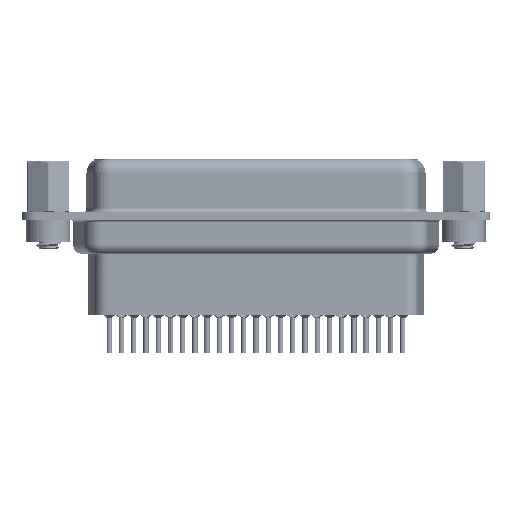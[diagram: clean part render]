
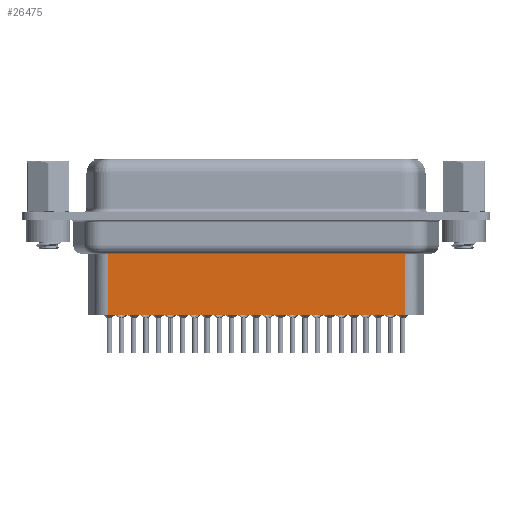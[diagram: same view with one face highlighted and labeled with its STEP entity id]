
A CAD part, front view. The second image highlights one B-rep face of the part: STEP entity #26475.
In plain terms, the highlighted planar face has unit normal (0, -1, 0).
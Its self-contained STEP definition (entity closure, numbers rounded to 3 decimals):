
#90 = CARTESIAN_POINT ( 'NONE',  ( 6.706, -3.5, -11.15 ) ) ;
#1557 = CARTESIAN_POINT ( 'NONE',  ( 6.706, -3.5, -3.1 ) ) ;
#2123 = LINE ( 'NONE', #7905, #11021 ) ;
#3071 = VECTOR ( 'NONE', #17312, 1000. ) ;
#3142 = CARTESIAN_POINT ( 'NONE',  ( 6.706, -3.5, -11.15 ) ) ;
#3190 = DIRECTION ( 'NONE',  ( 0., -1., 0. ) ) ;
#3309 = DIRECTION ( 'NONE',  ( -1., 0., 0. ) ) ;
#5667 = FACE_OUTER_BOUND ( 'NONE', #26028, .T. ) ;
#6197 = AXIS2_PLACEMENT_3D ( 'NONE', #15733, #3190, #30944 ) ;
#6871 = ORIENTED_EDGE ( 'NONE', *, *, #12112, .F. ) ;
#7106 = LINE ( 'NONE', #20107, #3071 ) ;
#7382 = VECTOR ( 'NONE', #3309, 1000. ) ;
#7905 = CARTESIAN_POINT ( 'NONE',  ( 40.344, -3.5, -3.1 ) ) ;
#8128 = EDGE_CURVE ( 'NONE', #25138, #25319, #2123, .T. ) ;
#8270 = CARTESIAN_POINT ( 'NONE',  ( 40.344, -3.5, -4.097 ) ) ;
#10207 = DIRECTION ( 'NONE',  ( 0., 0., -1. ) ) ;
#11021 = VECTOR ( 'NONE', #10207, 1000. ) ;
#11253 = CARTESIAN_POINT ( 'NONE',  ( 6.706, -3.5, -4.097 ) ) ;
#11737 = ORIENTED_EDGE ( 'NONE', *, *, #8128, .F. ) ;
#12112 = EDGE_CURVE ( 'NONE', #25319, #20810, #25782, .T. ) ;
#12355 = EDGE_CURVE ( 'NONE', #25138, #28070, #7106, .T. ) ;
#12894 = ORIENTED_EDGE ( 'NONE', *, *, #22030, .T. ) ;
#14116 = LINE ( 'NONE', #1557, #18735 ) ;
#15733 = CARTESIAN_POINT ( 'NONE',  ( 6.706, -3.5, -3.1 ) ) ;
#17312 = DIRECTION ( 'NONE',  ( -1., 0., 0. ) ) ;
#18735 = VECTOR ( 'NONE', #23885, 1000. ) ;
#19384 = ORIENTED_EDGE ( 'NONE', *, *, #12355, .T. ) ;
#20107 = CARTESIAN_POINT ( 'NONE',  ( 6.459, -3.5, -4.097 ) ) ;
#20810 = VERTEX_POINT ( 'NONE', #90 ) ;
#22030 = EDGE_CURVE ( 'NONE', #28070, #20810, #14116, .T. ) ;
#23172 = PLANE ( 'NONE',  #6197 ) ;
#23885 = DIRECTION ( 'NONE',  ( 0., 0., -1. ) ) ;
#25138 = VERTEX_POINT ( 'NONE', #8270 ) ;
#25319 = VERTEX_POINT ( 'NONE', #30037 ) ;
#25782 = LINE ( 'NONE', #3142, #7382 ) ;
#26028 = EDGE_LOOP ( 'NONE', ( #11737, #19384, #12894, #6871 ) ) ;
#26475 = ADVANCED_FACE ( 'NONE', ( #5667 ), #23172, .T. ) ;
#28070 = VERTEX_POINT ( 'NONE', #11253 ) ;
#30037 = CARTESIAN_POINT ( 'NONE',  ( 40.344, -3.5, -11.15 ) ) ;
#30944 = DIRECTION ( 'NONE',  ( 1., 0., 0. ) ) ;
